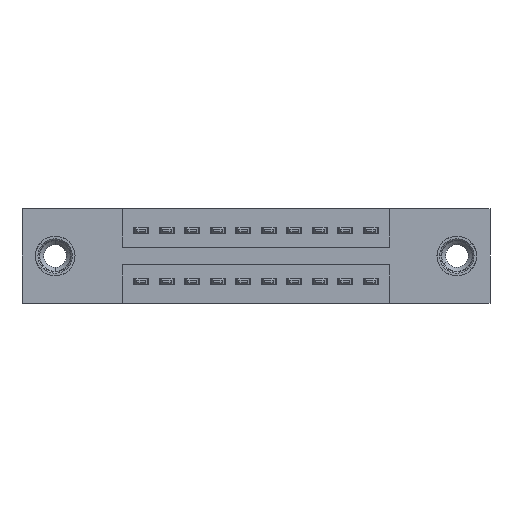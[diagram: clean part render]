
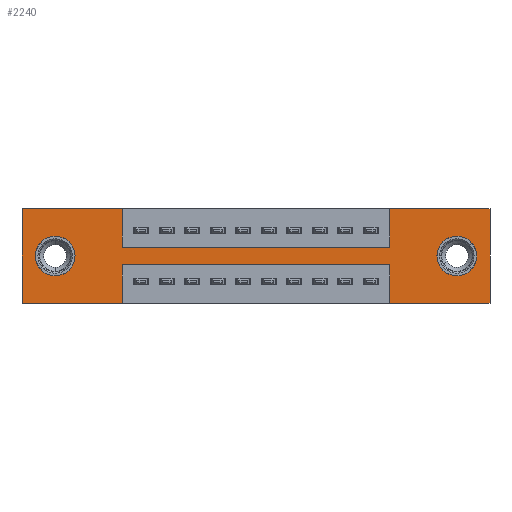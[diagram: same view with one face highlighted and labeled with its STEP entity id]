
A CAD part, front view. The second image highlights one B-rep face of the part: STEP entity #2240.
In plain terms, the highlighted planar face has unit normal (0, -1, 0).
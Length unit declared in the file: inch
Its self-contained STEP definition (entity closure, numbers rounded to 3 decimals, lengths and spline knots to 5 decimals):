
#3 = PLANE ( 'NONE',  #8291 ) ;
#165 = AXIS2_PLACEMENT_3D ( 'NONE', #2576, #5583, #7698 ) ;
#184 = ORIENTED_EDGE ( 'NONE', *, *, #4160, .F. ) ;
#238 = ORIENTED_EDGE ( 'NONE', *, *, #2544, .F. ) ;
#253 = DIRECTION ( 'NONE',  ( 0., 0., -1. ) ) ;
#265 = VERTEX_POINT ( 'NONE', #12189 ) ;
#348 = CARTESIAN_POINT ( 'NONE',  ( 1.705, 0., -0.185 ) ) ;
#741 = VECTOR ( 'NONE', #4747, 39.37008 ) ;
#862 = CARTESIAN_POINT ( 'NONE',  ( 0., 0., -0.37 ) ) ;
#1169 = CARTESIAN_POINT ( 'NONE',  ( 0.3925, 0., -0.15 ) ) ;
#1246 = DIRECTION ( 'NONE',  ( 0., 1., 0. ) ) ;
#1537 = EDGE_CURVE ( 'NONE', #5877, #6197, #4838, .T. ) ;
#1602 = ORIENTED_EDGE ( 'NONE', *, *, #5301, .T. ) ;
#1743 = EDGE_CURVE ( 'NONE', #12699, #7801, #6245, .T. ) ;
#1902 = CARTESIAN_POINT ( 'NONE',  ( 0.3925, 0., -0.37 ) ) ;
#1921 = LINE ( 'NONE', #11666, #6804 ) ;
#2144 = FACE_OUTER_BOUND ( 'NONE', #8947, .T. ) ;
#2240 = ADVANCED_FACE ( 'NONE', ( #7033, #3538, #2144 ), #3, .T. ) ;
#2347 = DIRECTION ( 'NONE',  ( 0., 0., 1. ) ) ;
#2461 = CARTESIAN_POINT ( 'NONE',  ( 0.3925, 0., 0. ) ) ;
#2543 = ORIENTED_EDGE ( 'NONE', *, *, #5136, .T. ) ;
#2544 = EDGE_CURVE ( 'NONE', #9698, #8703, #5405, .T. ) ;
#2576 = CARTESIAN_POINT ( 'NONE',  ( 0.13, 0., -0.185 ) ) ;
#2691 = CIRCLE ( 'NONE', #10157, 0.078 ) ;
#2835 = DIRECTION ( 'NONE',  ( 0., 0., 1. ) ) ;
#3038 = CARTESIAN_POINT ( 'NONE',  ( 0., 0., -0.37 ) ) ;
#3169 = CARTESIAN_POINT ( 'NONE',  ( 1.4425, 0., -0.22 ) ) ;
#3466 = CARTESIAN_POINT ( 'NONE',  ( 1.4425, 0., 0. ) ) ;
#3538 = FACE_BOUND ( 'NONE', #8667, .T. ) ;
#3767 = VERTEX_POINT ( 'NONE', #11471 ) ;
#3773 = CIRCLE ( 'NONE', #4802, 0.078 ) ;
#3844 = CARTESIAN_POINT ( 'NONE',  ( 0.3925, 0., 0. ) ) ;
#3856 = VERTEX_POINT ( 'NONE', #7279 ) ;
#3863 = VERTEX_POINT ( 'NONE', #3169 ) ;
#3932 = ORIENTED_EDGE ( 'NONE', *, *, #11347, .F. ) ;
#4019 = CARTESIAN_POINT ( 'NONE',  ( 0.3925, 0., -0.22 ) ) ;
#4160 = EDGE_CURVE ( 'NONE', #9787, #9698, #10088, .T. ) ;
#4172 = DIRECTION ( 'NONE',  ( 0., 0., -1. ) ) ;
#4693 = CARTESIAN_POINT ( 'NONE',  ( 1.4425, 0., -0.15 ) ) ;
#4747 = DIRECTION ( 'NONE',  ( -1., 0., 0. ) ) ;
#4802 = AXIS2_PLACEMENT_3D ( 'NONE', #5971, #1246, #8006 ) ;
#4806 = VECTOR ( 'NONE', #2835, 39.37008 ) ;
#4838 = CIRCLE ( 'NONE', #5176, 0.078 ) ;
#4994 = EDGE_CURVE ( 'NONE', #5489, #8356, #7545, .T. ) ;
#5011 = ORIENTED_EDGE ( 'NONE', *, *, #6516, .F. ) ;
#5044 = DIRECTION ( 'NONE',  ( -1., 0., 0. ) ) ;
#5136 = EDGE_CURVE ( 'NONE', #6197, #5877, #2691, .T. ) ;
#5176 = AXIS2_PLACEMENT_3D ( 'NONE', #348, #8364, #253 ) ;
#5226 = DIRECTION ( 'NONE',  ( 1., 0., 0. ) ) ;
#5235 = DIRECTION ( 'NONE',  ( 0., 0., -1. ) ) ;
#5301 = EDGE_CURVE ( 'NONE', #3856, #3767, #3773, .T. ) ;
#5350 = DIRECTION ( 'NONE',  ( 0., 0., -1. ) ) ;
#5405 = LINE ( 'NONE', #2461, #7172 ) ;
#5489 = VERTEX_POINT ( 'NONE', #4693 ) ;
#5568 = ORIENTED_EDGE ( 'NONE', *, *, #1537, .T. ) ;
#5583 = DIRECTION ( 'NONE',  ( 0., 1., 0. ) ) ;
#5589 = LINE ( 'NONE', #9246, #7866 ) ;
#5806 = DIRECTION ( 'NONE',  ( 1., 0., 0. ) ) ;
#5819 = CARTESIAN_POINT ( 'NONE',  ( 0., 0., 0. ) ) ;
#5829 = VERTEX_POINT ( 'NONE', #8190 ) ;
#5848 = CARTESIAN_POINT ( 'NONE',  ( 1.4425, 0., -0.37 ) ) ;
#5877 = VERTEX_POINT ( 'NONE', #10462 ) ;
#5971 = CARTESIAN_POINT ( 'NONE',  ( 0.13, 0., -0.185 ) ) ;
#6061 = CARTESIAN_POINT ( 'NONE',  ( 0., 0., 0. ) ) ;
#6158 = EDGE_CURVE ( 'NONE', #6944, #9110, #7904, .T. ) ;
#6197 = VERTEX_POINT ( 'NONE', #8779 ) ;
#6245 = LINE ( 'NONE', #11829, #741 ) ;
#6391 = CIRCLE ( 'NONE', #165, 0.078 ) ;
#6474 = EDGE_LOOP ( 'NONE', ( #5568, #2543 ) ) ;
#6516 = EDGE_CURVE ( 'NONE', #3863, #5829, #9836, .T. ) ;
#6657 = CARTESIAN_POINT ( 'NONE',  ( 0., 0., -0.37 ) ) ;
#6804 = VECTOR ( 'NONE', #10170, 39.37008 ) ;
#6944 = VERTEX_POINT ( 'NONE', #8715 ) ;
#7032 = LINE ( 'NONE', #5848, #4806 ) ;
#7033 = FACE_BOUND ( 'NONE', #6474, .T. ) ;
#7050 = ORIENTED_EDGE ( 'NONE', *, *, #8044, .F. ) ;
#7172 = VECTOR ( 'NONE', #5350, 39.37008 ) ;
#7209 = VECTOR ( 'NONE', #2347, 39.37008 ) ;
#7279 = CARTESIAN_POINT ( 'NONE',  ( 0.13, 0., -0.263 ) ) ;
#7358 = LINE ( 'NONE', #12980, #7513 ) ;
#7367 = ORIENTED_EDGE ( 'NONE', *, *, #10862, .F. ) ;
#7457 = VECTOR ( 'NONE', #5226, 39.37008 ) ;
#7476 = VECTOR ( 'NONE', #11305, 39.37008 ) ;
#7513 = VECTOR ( 'NONE', #8945, 39.37008 ) ;
#7545 = LINE ( 'NONE', #3466, #7209 ) ;
#7649 = DIRECTION ( 'NONE',  ( 0., 1., 0. ) ) ;
#7693 = DIRECTION ( 'NONE',  ( -1., 0., 0. ) ) ;
#7698 = DIRECTION ( 'NONE',  ( 0., 0., 1. ) ) ;
#7801 = VERTEX_POINT ( 'NONE', #862 ) ;
#7817 = LINE ( 'NONE', #9240, #7476 ) ;
#7828 = ORIENTED_EDGE ( 'NONE', *, *, #1743, .F. ) ;
#7866 = VECTOR ( 'NONE', #5235, 39.37008 ) ;
#7904 = LINE ( 'NONE', #6657, #12718 ) ;
#8006 = DIRECTION ( 'NONE',  ( 0., 0., 1. ) ) ;
#8044 = EDGE_CURVE ( 'NONE', #265, #6944, #5589, .T. ) ;
#8190 = CARTESIAN_POINT ( 'NONE',  ( 0.3925, 0., -0.22 ) ) ;
#8291 = AXIS2_PLACEMENT_3D ( 'NONE', #3038, #10378, #4172 ) ;
#8356 = VERTEX_POINT ( 'NONE', #9509 ) ;
#8364 = DIRECTION ( 'NONE',  ( 0., 1., 0. ) ) ;
#8493 = EDGE_CURVE ( 'NONE', #3767, #3856, #6391, .T. ) ;
#8503 = ORIENTED_EDGE ( 'NONE', *, *, #10010, .F. ) ;
#8596 = CARTESIAN_POINT ( 'NONE',  ( 1.705, 0., -0.185 ) ) ;
#8667 = EDGE_LOOP ( 'NONE', ( #12866, #1602 ) ) ;
#8703 = VERTEX_POINT ( 'NONE', #1169 ) ;
#8715 = CARTESIAN_POINT ( 'NONE',  ( 1.835, 0., -0.37 ) ) ;
#8779 = CARTESIAN_POINT ( 'NONE',  ( 1.705, 0., -0.263 ) ) ;
#8945 = DIRECTION ( 'NONE',  ( 1., 0., 0. ) ) ;
#8947 = EDGE_LOOP ( 'NONE', ( #7367, #5011, #13143, #12949, #7050, #3932, #11678, #10198, #238, #184, #8503, #7828 ) ) ;
#9110 = VERTEX_POINT ( 'NONE', #10850 ) ;
#9240 = CARTESIAN_POINT ( 'NONE',  ( 0., 0., 0. ) ) ;
#9246 = CARTESIAN_POINT ( 'NONE',  ( 1.835, 0., 0. ) ) ;
#9509 = CARTESIAN_POINT ( 'NONE',  ( 1.4425, 0., 0. ) ) ;
#9698 = VERTEX_POINT ( 'NONE', #3844 ) ;
#9787 = VERTEX_POINT ( 'NONE', #5819 ) ;
#9836 = LINE ( 'NONE', #4019, #11109 ) ;
#10010 = EDGE_CURVE ( 'NONE', #7801, #9787, #7817, .T. ) ;
#10088 = LINE ( 'NONE', #11399, #7457 ) ;
#10157 = AXIS2_PLACEMENT_3D ( 'NONE', #8596, #7649, #10768 ) ;
#10170 = DIRECTION ( 'NONE',  ( 0., 0., -1. ) ) ;
#10198 = ORIENTED_EDGE ( 'NONE', *, *, #11900, .F. ) ;
#10378 = DIRECTION ( 'NONE',  ( 0., -1., 0. ) ) ;
#10462 = CARTESIAN_POINT ( 'NONE',  ( 1.705, 0., -0.107 ) ) ;
#10768 = DIRECTION ( 'NONE',  ( 0., 0., -1. ) ) ;
#10850 = CARTESIAN_POINT ( 'NONE',  ( 1.4425, 0., -0.37 ) ) ;
#10862 = EDGE_CURVE ( 'NONE', #5829, #12699, #1921, .T. ) ;
#11109 = VECTOR ( 'NONE', #5044, 39.37008 ) ;
#11305 = DIRECTION ( 'NONE',  ( 0., 0., 1. ) ) ;
#11347 = EDGE_CURVE ( 'NONE', #8356, #265, #13062, .T. ) ;
#11399 = CARTESIAN_POINT ( 'NONE',  ( 0., 0., 0. ) ) ;
#11471 = CARTESIAN_POINT ( 'NONE',  ( 0.13, 0., -0.107 ) ) ;
#11625 = EDGE_CURVE ( 'NONE', #9110, #3863, #7032, .T. ) ;
#11666 = CARTESIAN_POINT ( 'NONE',  ( 0.3925, 0., -0.37 ) ) ;
#11678 = ORIENTED_EDGE ( 'NONE', *, *, #4994, .F. ) ;
#11829 = CARTESIAN_POINT ( 'NONE',  ( 0., 0., -0.37 ) ) ;
#11900 = EDGE_CURVE ( 'NONE', #8703, #5489, #7358, .T. ) ;
#12189 = CARTESIAN_POINT ( 'NONE',  ( 1.835, 0., 0. ) ) ;
#12581 = VECTOR ( 'NONE', #5806, 39.37008 ) ;
#12699 = VERTEX_POINT ( 'NONE', #1902 ) ;
#12718 = VECTOR ( 'NONE', #7693, 39.37008 ) ;
#12866 = ORIENTED_EDGE ( 'NONE', *, *, #8493, .T. ) ;
#12949 = ORIENTED_EDGE ( 'NONE', *, *, #6158, .F. ) ;
#12980 = CARTESIAN_POINT ( 'NONE',  ( 0.3925, 0., -0.15 ) ) ;
#13062 = LINE ( 'NONE', #6061, #12581 ) ;
#13143 = ORIENTED_EDGE ( 'NONE', *, *, #11625, .F. ) ;
